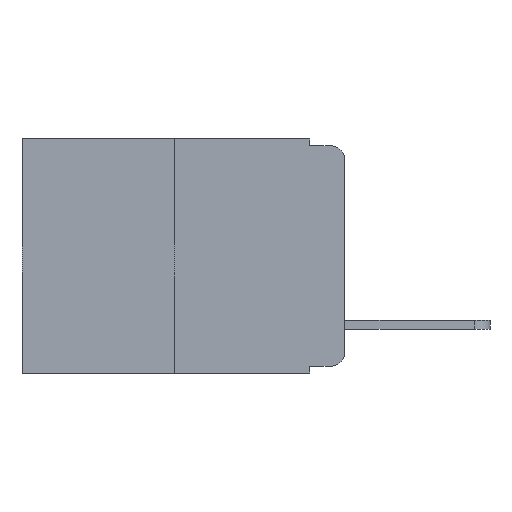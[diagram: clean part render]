
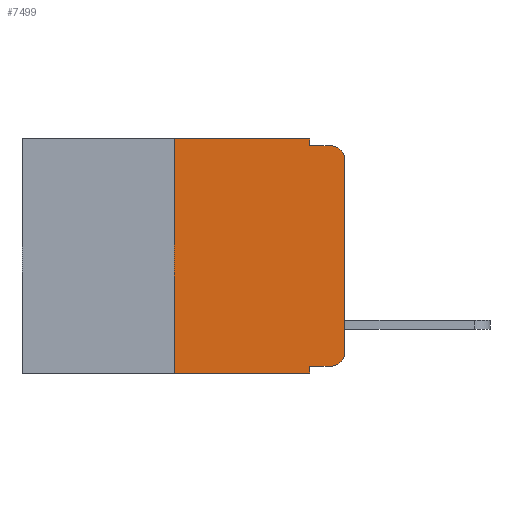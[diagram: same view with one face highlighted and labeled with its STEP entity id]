
A CAD part, left-side view. The second image highlights one B-rep face of the part: STEP entity #7499.
In plain terms, the highlighted planar face has unit normal (-1, 0, 0).
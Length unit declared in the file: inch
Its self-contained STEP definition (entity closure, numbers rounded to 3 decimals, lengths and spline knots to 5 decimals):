
#16 = LINE ( 'NONE', #8240, #2484 ) ;
#34 = CARTESIAN_POINT ( 'NONE',  ( 0., 0.473, 0. ) ) ;
#87 = VECTOR ( 'NONE', #324, 39.37008 ) ;
#159 = CARTESIAN_POINT ( 'NONE',  ( 0., 0.02, -0.01 ) ) ;
#324 = DIRECTION ( 'NONE',  ( 0., 0., 1. ) ) ;
#335 = LINE ( 'NONE', #4084, #4296 ) ;
#414 = LINE ( 'NONE', #11917, #87 ) ;
#1046 = ORIENTED_EDGE ( 'NONE', *, *, #1089, .F. ) ;
#1054 = VERTEX_POINT ( 'NONE', #2870 ) ;
#1089 = EDGE_CURVE ( 'NONE', #11454, #1337, #6499, .T. ) ;
#1319 = CIRCLE ( 'NONE', #12995, 0.02 ) ;
#1337 = VERTEX_POINT ( 'NONE', #11062 ) ;
#1414 = VECTOR ( 'NONE', #13455, 39.37008 ) ;
#1775 = ORIENTED_EDGE ( 'NONE', *, *, #7489, .F. ) ;
#1789 = CARTESIAN_POINT ( 'NONE',  ( 0., 0.051, -0.343 ) ) ;
#2017 = DIRECTION ( 'NONE',  ( 0., 0., -1. ) ) ;
#2411 = ORIENTED_EDGE ( 'NONE', *, *, #8389, .T. ) ;
#2440 = CARTESIAN_POINT ( 'NONE',  ( 0., 0., 0. ) ) ;
#2484 = VECTOR ( 'NONE', #4049, 39.37008 ) ;
#2617 = LINE ( 'NONE', #2440, #9404 ) ;
#2668 = ORIENTED_EDGE ( 'NONE', *, *, #12563, .T. ) ;
#2814 = VECTOR ( 'NONE', #5271, 39.37008 ) ;
#2817 = EDGE_LOOP ( 'NONE', ( #2411, #11008, #3914, #1775, #1046, #5523, #2668, #9857, #3762, #9775 ) ) ;
#2837 = CARTESIAN_POINT ( 'NONE',  ( 0., 0.051, -0.01 ) ) ;
#2857 = CIRCLE ( 'NONE', #8674, 0.02 ) ;
#2870 = CARTESIAN_POINT ( 'NONE',  ( 0., 0., -0.03 ) ) ;
#3379 = VERTEX_POINT ( 'NONE', #2837 ) ;
#3628 = VERTEX_POINT ( 'NONE', #10853 ) ;
#3762 = ORIENTED_EDGE ( 'NONE', *, *, #6688, .T. ) ;
#3813 = LINE ( 'NONE', #7210, #8783 ) ;
#3914 = ORIENTED_EDGE ( 'NONE', *, *, #4686, .F. ) ;
#4049 = DIRECTION ( 'NONE',  ( 0., -1., 0. ) ) ;
#4054 = LINE ( 'NONE', #5102, #11998 ) ;
#4084 = CARTESIAN_POINT ( 'NONE',  ( 0., 0.051, 0. ) ) ;
#4296 = VECTOR ( 'NONE', #2017, 39.37008 ) ;
#4635 = EDGE_CURVE ( 'NONE', #12537, #6725, #9539, .T. ) ;
#4686 = EDGE_CURVE ( 'NONE', #3379, #13271, #4054, .T. ) ;
#5037 = CARTESIAN_POINT ( 'NONE',  ( 0., 0.051, -0.333 ) ) ;
#5044 = EDGE_CURVE ( 'NONE', #5359, #11454, #414, .T. ) ;
#5102 = CARTESIAN_POINT ( 'NONE',  ( 0., 0.051, -0.01 ) ) ;
#5182 = DIRECTION ( 'NONE',  ( 0., -1., 0. ) ) ;
#5271 = DIRECTION ( 'NONE',  ( 0., -1., 0. ) ) ;
#5277 = DIRECTION ( 'NONE',  ( -1., 0., 0. ) ) ;
#5359 = VERTEX_POINT ( 'NONE', #6104 ) ;
#5523 = ORIENTED_EDGE ( 'NONE', *, *, #5044, .F. ) ;
#6104 = CARTESIAN_POINT ( 'NONE',  ( 0., 0.25, -0.343 ) ) ;
#6120 = CARTESIAN_POINT ( 'NONE',  ( 0., 0.051, 0. ) ) ;
#6499 = LINE ( 'NONE', #34, #2814 ) ;
#6688 = EDGE_CURVE ( 'NONE', #12537, #10894, #16, .T. ) ;
#6725 = VERTEX_POINT ( 'NONE', #1789 ) ;
#6909 = DIRECTION ( 'NONE',  ( -1., 0., 0. ) ) ;
#7039 = CARTESIAN_POINT ( 'NONE',  ( 0., 0.02, -0.313 ) ) ;
#7210 = CARTESIAN_POINT ( 'NONE',  ( 0., 0.473, -0.343 ) ) ;
#7489 = EDGE_CURVE ( 'NONE', #1337, #3379, #335, .T. ) ;
#7499 = ADVANCED_FACE ( 'NONE', ( #13049 ), #11516, .F. ) ;
#7951 = EDGE_CURVE ( 'NONE', #10894, #3628, #1319, .T. ) ;
#8240 = CARTESIAN_POINT ( 'NONE',  ( 0., 0.051, -0.333 ) ) ;
#8389 = EDGE_CURVE ( 'NONE', #3628, #1054, #2617, .T. ) ;
#8568 = AXIS2_PLACEMENT_3D ( 'NONE', #12592, #12493, #13556 ) ;
#8674 = AXIS2_PLACEMENT_3D ( 'NONE', #9523, #5277, #11710 ) ;
#8783 = VECTOR ( 'NONE', #5182, 39.37008 ) ;
#8900 = EDGE_CURVE ( 'NONE', #1054, #13271, #2857, .T. ) ;
#9404 = VECTOR ( 'NONE', #10867, 39.37008 ) ;
#9523 = CARTESIAN_POINT ( 'NONE',  ( 0., 0.02, -0.03 ) ) ;
#9539 = LINE ( 'NONE', #6120, #1414 ) ;
#9775 = ORIENTED_EDGE ( 'NONE', *, *, #7951, .T. ) ;
#9857 = ORIENTED_EDGE ( 'NONE', *, *, #4635, .F. ) ;
#9910 = CARTESIAN_POINT ( 'NONE',  ( 0., 0.25, 0. ) ) ;
#10142 = DIRECTION ( 'NONE',  ( 0., 0., -1. ) ) ;
#10853 = CARTESIAN_POINT ( 'NONE',  ( 0., 0., -0.313 ) ) ;
#10867 = DIRECTION ( 'NONE',  ( 0., 0., 1. ) ) ;
#10894 = VERTEX_POINT ( 'NONE', #11792 ) ;
#11008 = ORIENTED_EDGE ( 'NONE', *, *, #8900, .T. ) ;
#11062 = CARTESIAN_POINT ( 'NONE',  ( 0., 0.051, 0. ) ) ;
#11454 = VERTEX_POINT ( 'NONE', #9910 ) ;
#11516 = PLANE ( 'NONE',  #8568 ) ;
#11710 = DIRECTION ( 'NONE',  ( 0., 0., -1. ) ) ;
#11792 = CARTESIAN_POINT ( 'NONE',  ( 0., 0.02, -0.333 ) ) ;
#11917 = CARTESIAN_POINT ( 'NONE',  ( 0., 0.25, 0. ) ) ;
#11998 = VECTOR ( 'NONE', #13635, 39.37008 ) ;
#12493 = DIRECTION ( 'NONE',  ( 1., 0., 0. ) ) ;
#12537 = VERTEX_POINT ( 'NONE', #5037 ) ;
#12563 = EDGE_CURVE ( 'NONE', #5359, #6725, #3813, .T. ) ;
#12592 = CARTESIAN_POINT ( 'NONE',  ( 0., 0.473, 0. ) ) ;
#12995 = AXIS2_PLACEMENT_3D ( 'NONE', #7039, #6909, #10142 ) ;
#13049 = FACE_OUTER_BOUND ( 'NONE', #2817, .T. ) ;
#13271 = VERTEX_POINT ( 'NONE', #159 ) ;
#13455 = DIRECTION ( 'NONE',  ( 0., 0., -1. ) ) ;
#13556 = DIRECTION ( 'NONE',  ( 0., 0., -1. ) ) ;
#13635 = DIRECTION ( 'NONE',  ( 0., -1., 0. ) ) ;
